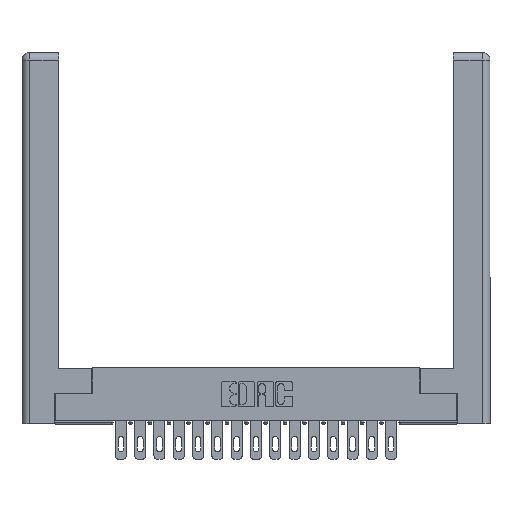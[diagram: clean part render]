
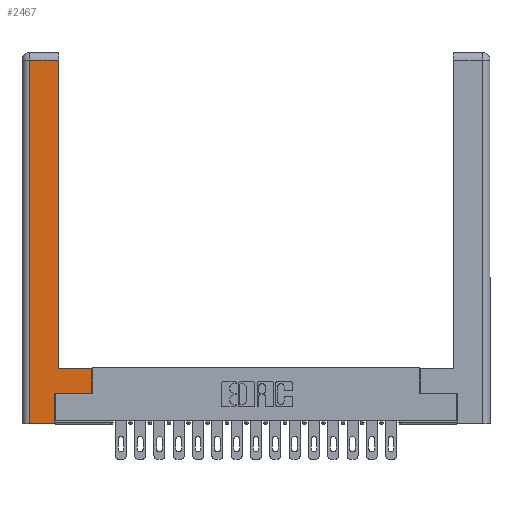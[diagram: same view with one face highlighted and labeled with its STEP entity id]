
A CAD part, top view. The second image highlights one B-rep face of the part: STEP entity #2467.
In plain terms, the highlighted planar face has unit normal (0, 0, 1).
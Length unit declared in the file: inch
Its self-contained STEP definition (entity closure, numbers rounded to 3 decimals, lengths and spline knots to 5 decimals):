
#1582 = VECTOR ( 'NONE', #5044, 39.37008 ) ;
#1919 = EDGE_LOOP ( 'NONE', ( #11183, #19088, #16971, #14549, #19735, #3768, #13355, #3537 ) ) ;
#2364 = EDGE_CURVE ( 'NONE', #6549, #2410, #13838, .T. ) ;
#2410 = VERTEX_POINT ( 'NONE', #11831 ) ;
#2467 = ADVANCED_FACE ( 'NONE', ( #18939 ), #19476, .F. ) ;
#2833 = EDGE_CURVE ( 'NONE', #10810, #14613, #8688, .T. ) ;
#3319 = CARTESIAN_POINT ( 'NONE',  ( 0.565, 0.45, 0. ) ) ;
#3537 = ORIENTED_EDGE ( 'NONE', *, *, #11466, .T. ) ;
#3768 = ORIENTED_EDGE ( 'NONE', *, *, #12709, .T. ) ;
#4222 = VERTEX_POINT ( 'NONE', #5712 ) ;
#4591 = LINE ( 'NONE', #19737, #9359 ) ;
#5044 = DIRECTION ( 'NONE',  ( -1., 0., 0. ) ) ;
#5287 = VECTOR ( 'NONE', #6733, 39.37008 ) ;
#5712 = CARTESIAN_POINT ( 'NONE',  ( 0.295, 0.45, 0. ) ) ;
#6120 = LINE ( 'NONE', #18709, #1582 ) ;
#6202 = LINE ( 'NONE', #12936, #21725 ) ;
#6276 = DIRECTION ( 'NONE',  ( -1., 0., 0. ) ) ;
#6549 = VERTEX_POINT ( 'NONE', #20152 ) ;
#6733 = DIRECTION ( 'NONE',  ( 0., 1., 0. ) ) ;
#7539 = EDGE_CURVE ( 'NONE', #16153, #13789, #19325, .T. ) ;
#8688 = LINE ( 'NONE', #3319, #5287 ) ;
#9202 = DIRECTION ( 'NONE',  ( 0., 0., -1. ) ) ;
#9345 = CARTESIAN_POINT ( 'NONE',  ( 0., 0., 0. ) ) ;
#9359 = VECTOR ( 'NONE', #9466, 39.37008 ) ;
#9466 = DIRECTION ( 'NONE',  ( 0., 1., 0. ) ) ;
#9555 = CARTESIAN_POINT ( 'NONE',  ( 0.265, 0.245, 0. ) ) ;
#9630 = CARTESIAN_POINT ( 'NONE',  ( 0.295, 0.45, 0. ) ) ;
#9970 = DIRECTION ( 'NONE',  ( 0., -1., 0. ) ) ;
#10062 = LINE ( 'NONE', #18824, #11119 ) ;
#10357 = CARTESIAN_POINT ( 'NONE',  ( 0.565, 0.245, 0. ) ) ;
#10810 = VERTEX_POINT ( 'NONE', #10357 ) ;
#11119 = VECTOR ( 'NONE', #22128, 39.37008 ) ;
#11183 = ORIENTED_EDGE ( 'NONE', *, *, #20233, .T. ) ;
#11466 = EDGE_CURVE ( 'NONE', #14613, #4222, #11588, .T. ) ;
#11588 = LINE ( 'NONE', #9630, #15652 ) ;
#11831 = CARTESIAN_POINT ( 'NONE',  ( 0.0615, 0., 0. ) ) ;
#12709 = EDGE_CURVE ( 'NONE', #13789, #10810, #10062, .T. ) ;
#12936 = CARTESIAN_POINT ( 'NONE',  ( 0.265, 0., 0. ) ) ;
#13355 = ORIENTED_EDGE ( 'NONE', *, *, #2833, .T. ) ;
#13789 = VERTEX_POINT ( 'NONE', #20883 ) ;
#13838 = LINE ( 'NONE', #20391, #14916 ) ;
#14505 = DIRECTION ( 'NONE',  ( 0., 1., 0. ) ) ;
#14549 = ORIENTED_EDGE ( 'NONE', *, *, #15289, .T. ) ;
#14613 = VERTEX_POINT ( 'NONE', #15477 ) ;
#14848 = CARTESIAN_POINT ( 'NONE',  ( 0.265, 0., 0. ) ) ;
#14916 = VECTOR ( 'NONE', #9970, 39.37008 ) ;
#15053 = CARTESIAN_POINT ( 'NONE',  ( 0.295, 2.94, 0. ) ) ;
#15289 = EDGE_CURVE ( 'NONE', #2410, #16153, #6202, .T. ) ;
#15477 = CARTESIAN_POINT ( 'NONE',  ( 0.565, 0.45, 0. ) ) ;
#15652 = VECTOR ( 'NONE', #6276, 39.37008 ) ;
#16153 = VERTEX_POINT ( 'NONE', #14848 ) ;
#16638 = VECTOR ( 'NONE', #14505, 39.37008 ) ;
#16930 = EDGE_CURVE ( 'NONE', #18600, #6549, #6120, .T. ) ;
#16971 = ORIENTED_EDGE ( 'NONE', *, *, #2364, .T. ) ;
#18600 = VERTEX_POINT ( 'NONE', #15053 ) ;
#18709 = CARTESIAN_POINT ( 'NONE',  ( 0.0615, 2.94, 0. ) ) ;
#18824 = CARTESIAN_POINT ( 'NONE',  ( 0.565, 0.245, 0. ) ) ;
#18939 = FACE_OUTER_BOUND ( 'NONE', #1919, .T. ) ;
#19088 = ORIENTED_EDGE ( 'NONE', *, *, #16930, .T. ) ;
#19325 = LINE ( 'NONE', #9555, #16638 ) ;
#19476 = PLANE ( 'NONE',  #19800 ) ;
#19735 = ORIENTED_EDGE ( 'NONE', *, *, #7539, .T. ) ;
#19737 = CARTESIAN_POINT ( 'NONE',  ( 0.295, 3., 0. ) ) ;
#19787 = DIRECTION ( 'NONE',  ( 1., 0., 0. ) ) ;
#19800 = AXIS2_PLACEMENT_3D ( 'NONE', #9345, #9202, #21351 ) ;
#20152 = CARTESIAN_POINT ( 'NONE',  ( 0.0615, 2.94, 0. ) ) ;
#20233 = EDGE_CURVE ( 'NONE', #4222, #18600, #4591, .T. ) ;
#20391 = CARTESIAN_POINT ( 'NONE',  ( 0.0615, 0., 0. ) ) ;
#20883 = CARTESIAN_POINT ( 'NONE',  ( 0.265, 0.245, 0. ) ) ;
#21351 = DIRECTION ( 'NONE',  ( -1., 0., 0. ) ) ;
#21725 = VECTOR ( 'NONE', #19787, 39.37008 ) ;
#22128 = DIRECTION ( 'NONE',  ( 1., 0., 0. ) ) ;
